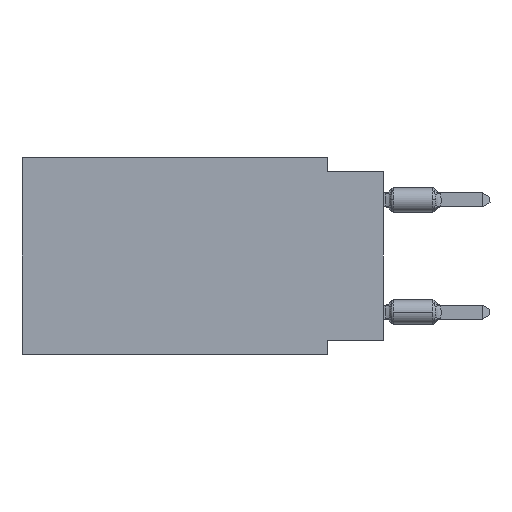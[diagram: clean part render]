
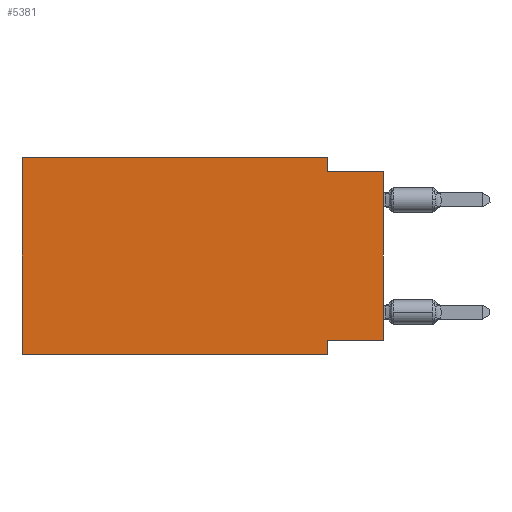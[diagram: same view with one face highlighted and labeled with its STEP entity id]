
A CAD part, left-side view. The second image highlights one B-rep face of the part: STEP entity #5381.
In plain terms, the highlighted planar face has unit normal (-1, 0, 0).
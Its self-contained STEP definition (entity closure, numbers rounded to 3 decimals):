
#231 = ORIENTED_EDGE ( 'NONE', *, *, #11645, .F. ) ;
#360 = LINE ( 'NONE', #3967, #8017 ) ;
#435 = LINE ( 'NONE', #4121, #14128 ) ;
#521 = CARTESIAN_POINT ( 'NONE',  ( 0., 2.54, -0.635 ) ) ;
#1200 = DIRECTION ( 'NONE',  ( 0., 0., -1. ) ) ;
#1284 = DIRECTION ( 'NONE',  ( 0., -1., 0. ) ) ;
#1347 = EDGE_CURVE ( 'NONE', #12832, #13036, #14134, .T. ) ;
#1476 = CARTESIAN_POINT ( 'NONE',  ( 0., 16.383, 0. ) ) ;
#1569 = EDGE_CURVE ( 'NONE', #5986, #10081, #8628, .T. ) ;
#2076 = EDGE_CURVE ( 'NONE', #12832, #5986, #360, .T. ) ;
#2703 = VECTOR ( 'NONE', #9231, 1000. ) ;
#2866 = DIRECTION ( 'NONE',  ( 0., 0., 1. ) ) ;
#3635 = VERTEX_POINT ( 'NONE', #13146 ) ;
#3967 = CARTESIAN_POINT ( 'NONE',  ( 0., 16.383, 0. ) ) ;
#4121 = CARTESIAN_POINT ( 'NONE',  ( 0., 0., 0. ) ) ;
#4124 = DIRECTION ( 'NONE',  ( 0., 0., 1. ) ) ;
#4286 = CARTESIAN_POINT ( 'NONE',  ( 0., 2.54, -8.255 ) ) ;
#4311 = CARTESIAN_POINT ( 'NONE',  ( 0., 16.383, -8.89 ) ) ;
#4462 = CARTESIAN_POINT ( 'NONE',  ( 0., 2.54, -8.89 ) ) ;
#4510 = CARTESIAN_POINT ( 'NONE',  ( 0., 0., -0.635 ) ) ;
#4708 = EDGE_CURVE ( 'NONE', #11352, #13036, #6714, .T. ) ;
#4806 = FACE_OUTER_BOUND ( 'NONE', #12503, .T. ) ;
#5129 = VERTEX_POINT ( 'NONE', #521 ) ;
#5381 = ADVANCED_FACE ( 'NONE', ( #4806 ), #9675, .F. ) ;
#5632 = CARTESIAN_POINT ( 'NONE',  ( 0., 2.54, 0. ) ) ;
#5862 = LINE ( 'NONE', #5632, #13463 ) ;
#5916 = CARTESIAN_POINT ( 'NONE',  ( 0., 0., -8.255 ) ) ;
#5986 = VERTEX_POINT ( 'NONE', #14275 ) ;
#6265 = DIRECTION ( 'NONE',  ( 0., -1., 0. ) ) ;
#6296 = ORIENTED_EDGE ( 'NONE', *, *, #2076, .F. ) ;
#6444 = VERTEX_POINT ( 'NONE', #4510 ) ;
#6714 = LINE ( 'NONE', #13950, #2703 ) ;
#7085 = CARTESIAN_POINT ( 'NONE',  ( 0., 16.383, 0. ) ) ;
#7244 = CARTESIAN_POINT ( 'NONE',  ( 0., 0., -0.635 ) ) ;
#7816 = CARTESIAN_POINT ( 'NONE',  ( 0., 2.54, 0. ) ) ;
#8017 = VECTOR ( 'NONE', #4124, 1000. ) ;
#8141 = DIRECTION ( 'NONE',  ( 0., 0., -1. ) ) ;
#8426 = LINE ( 'NONE', #7244, #10764 ) ;
#8475 = AXIS2_PLACEMENT_3D ( 'NONE', #7085, #15498, #1200 ) ;
#8628 = LINE ( 'NONE', #1476, #9037 ) ;
#8773 = EDGE_CURVE ( 'NONE', #10081, #5129, #5862, .T. ) ;
#9037 = VECTOR ( 'NONE', #6265, 1000. ) ;
#9179 = CARTESIAN_POINT ( 'NONE',  ( 0., 16.383, -8.89 ) ) ;
#9231 = DIRECTION ( 'NONE',  ( 0., 0., -1. ) ) ;
#9526 = VECTOR ( 'NONE', #11779, 1000. ) ;
#9675 = PLANE ( 'NONE',  #8475 ) ;
#10081 = VERTEX_POINT ( 'NONE', #7816 ) ;
#10484 = DIRECTION ( 'NONE',  ( 0., 1., 0. ) ) ;
#10764 = VECTOR ( 'NONE', #1284, 1000. ) ;
#11288 = ORIENTED_EDGE ( 'NONE', *, *, #14864, .T. ) ;
#11352 = VERTEX_POINT ( 'NONE', #4286 ) ;
#11449 = EDGE_CURVE ( 'NONE', #3635, #11352, #15350, .T. ) ;
#11645 = EDGE_CURVE ( 'NONE', #5129, #6444, #8426, .T. ) ;
#11779 = DIRECTION ( 'NONE',  ( 0., -1., 0. ) ) ;
#12231 = ORIENTED_EDGE ( 'NONE', *, *, #1569, .F. ) ;
#12503 = EDGE_LOOP ( 'NONE', ( #11288, #231, #13807, #12231, #6296, #13285, #12743, #12685 ) ) ;
#12512 = VECTOR ( 'NONE', #10484, 1000. ) ;
#12685 = ORIENTED_EDGE ( 'NONE', *, *, #11449, .F. ) ;
#12743 = ORIENTED_EDGE ( 'NONE', *, *, #4708, .F. ) ;
#12832 = VERTEX_POINT ( 'NONE', #4311 ) ;
#13036 = VERTEX_POINT ( 'NONE', #4462 ) ;
#13146 = CARTESIAN_POINT ( 'NONE',  ( 0., 0., -8.255 ) ) ;
#13285 = ORIENTED_EDGE ( 'NONE', *, *, #1347, .T. ) ;
#13463 = VECTOR ( 'NONE', #8141, 1000. ) ;
#13807 = ORIENTED_EDGE ( 'NONE', *, *, #8773, .F. ) ;
#13950 = CARTESIAN_POINT ( 'NONE',  ( 0., 2.54, -8.89 ) ) ;
#14128 = VECTOR ( 'NONE', #2866, 1000. ) ;
#14134 = LINE ( 'NONE', #9179, #9526 ) ;
#14275 = CARTESIAN_POINT ( 'NONE',  ( 0., 16.383, 0. ) ) ;
#14864 = EDGE_CURVE ( 'NONE', #3635, #6444, #435, .T. ) ;
#15350 = LINE ( 'NONE', #5916, #12512 ) ;
#15498 = DIRECTION ( 'NONE',  ( 1., 0., 0. ) ) ;
